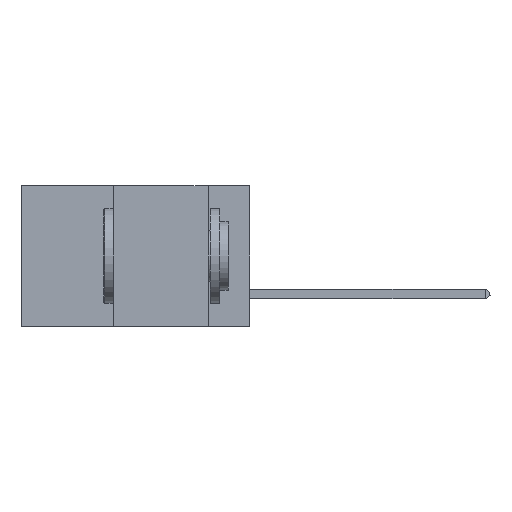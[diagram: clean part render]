
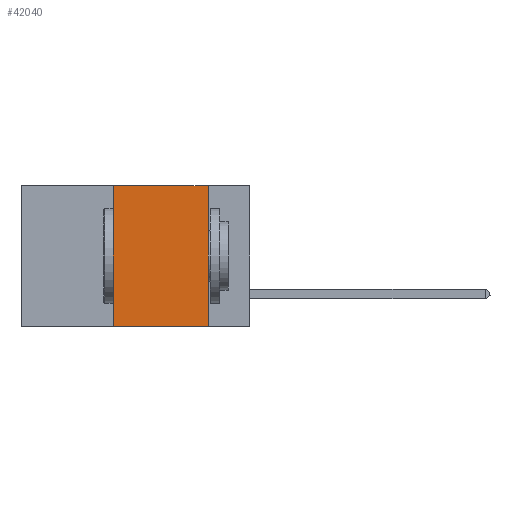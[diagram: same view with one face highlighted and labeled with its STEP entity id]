
A CAD part, left-side view. The second image highlights one B-rep face of the part: STEP entity #42040.
In plain terms, the highlighted planar face has unit normal (-1, 0, 0).
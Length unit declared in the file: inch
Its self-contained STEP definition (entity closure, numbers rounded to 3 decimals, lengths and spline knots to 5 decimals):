
#1042 = LINE ( 'NONE', #10441, #9826 ) ;
#1756 = VECTOR ( 'NONE', #15984, 39.37008 ) ;
#3048 = VERTEX_POINT ( 'NONE', #42187 ) ;
#3992 = DIRECTION ( 'NONE',  ( 0., -1., 0. ) ) ;
#4070 = CARTESIAN_POINT ( 'NONE',  ( 0., 0.36, -0.37 ) ) ;
#5803 = VECTOR ( 'NONE', #11506, 39.37008 ) ;
#9826 = VECTOR ( 'NONE', #14692, 39.37008 ) ;
#10441 = CARTESIAN_POINT ( 'NONE',  ( 0., 0.11, 0. ) ) ;
#10934 = EDGE_CURVE ( 'NONE', #19793, #21860, #1042, .T. ) ;
#11506 = DIRECTION ( 'NONE',  ( 0., -1., 0. ) ) ;
#11818 = CARTESIAN_POINT ( 'NONE',  ( 0., 0.6, -0.37 ) ) ;
#12058 = DIRECTION ( 'NONE',  ( 0., 0., -1. ) ) ;
#12235 = CARTESIAN_POINT ( 'NONE',  ( 0., 0.36, 0. ) ) ;
#14692 = DIRECTION ( 'NONE',  ( 0., 0., -1. ) ) ;
#14940 = CARTESIAN_POINT ( 'NONE',  ( 0., 0.6, 0. ) ) ;
#15984 = DIRECTION ( 'NONE',  ( 0., 0., 1. ) ) ;
#17715 = ORIENTED_EDGE ( 'NONE', *, *, #10934, .F. ) ;
#19491 = LINE ( 'NONE', #11818, #35374 ) ;
#19793 = VERTEX_POINT ( 'NONE', #23303 ) ;
#19820 = EDGE_CURVE ( 'NONE', #46545, #21860, #19491, .T. ) ;
#21860 = VERTEX_POINT ( 'NONE', #29294 ) ;
#23109 = ORIENTED_EDGE ( 'NONE', *, *, #24599, .F. ) ;
#23303 = CARTESIAN_POINT ( 'NONE',  ( 0., 0.11, 0. ) ) ;
#24599 = EDGE_CURVE ( 'NONE', #3048, #19793, #29847, .T. ) ;
#26028 = ORIENTED_EDGE ( 'NONE', *, *, #19820, .T. ) ;
#29294 = CARTESIAN_POINT ( 'NONE',  ( 0., 0.11, -0.37 ) ) ;
#29847 = LINE ( 'NONE', #14940, #5803 ) ;
#34198 = ORIENTED_EDGE ( 'NONE', *, *, #45465, .F. ) ;
#34625 = LINE ( 'NONE', #12235, #1756 ) ;
#35032 = FACE_OUTER_BOUND ( 'NONE', #41989, .T. ) ;
#35178 = AXIS2_PLACEMENT_3D ( 'NONE', #38790, #45650, #12058 ) ;
#35374 = VECTOR ( 'NONE', #3992, 39.37008 ) ;
#38790 = CARTESIAN_POINT ( 'NONE',  ( 0., 0.6, 0. ) ) ;
#41989 = EDGE_LOOP ( 'NONE', ( #17715, #23109, #34198, #26028 ) ) ;
#42040 = ADVANCED_FACE ( 'NONE', ( #35032 ), #42538, .F. ) ;
#42187 = CARTESIAN_POINT ( 'NONE',  ( 0., 0.36, 0. ) ) ;
#42538 = PLANE ( 'NONE',  #35178 ) ;
#45465 = EDGE_CURVE ( 'NONE', #46545, #3048, #34625, .T. ) ;
#45650 = DIRECTION ( 'NONE',  ( 1., 0., 0. ) ) ;
#46545 = VERTEX_POINT ( 'NONE', #4070 ) ;
